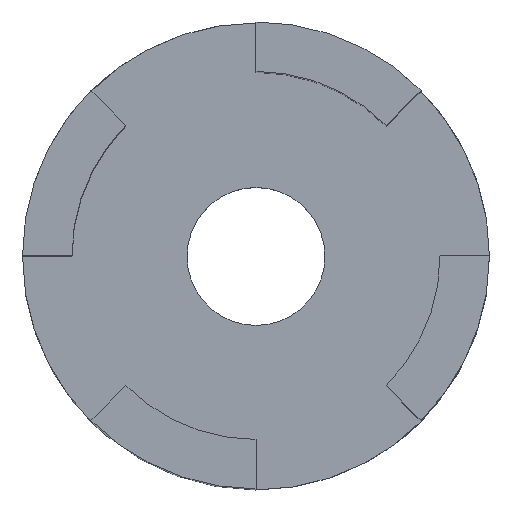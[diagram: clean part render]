
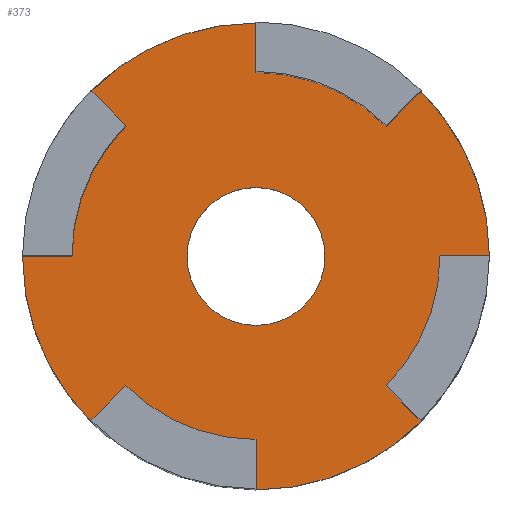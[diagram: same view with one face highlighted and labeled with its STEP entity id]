
A CAD part, top view. The second image highlights one B-rep face of the part: STEP entity #373.
In plain terms, the highlighted planar face has unit normal (0, 0, 1).
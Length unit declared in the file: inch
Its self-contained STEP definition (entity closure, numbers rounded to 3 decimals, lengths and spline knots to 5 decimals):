
#15=FACE_BOUND('',#65,.T.);
#26=PLANE('',#424);
#44=FACE_OUTER_BOUND('',#64,.T.);
#64=EDGE_LOOP('',(#300,#301,#302,#303,#304,#305,#306,#307,#308,#309,#310,
#311,#312,#313,#314,#315));
#65=EDGE_LOOP('',(#316));
#74=LINE('',#563,#108);
#79=LINE('',#577,#113);
#82=LINE('',#586,#116);
#87=LINE('',#600,#121);
#90=LINE('',#609,#124);
#95=LINE('',#623,#129);
#98=LINE('',#633,#132);
#99=LINE('',#637,#133);
#108=VECTOR('',#450,0.3937);
#113=VECTOR('',#463,0.3937);
#116=VECTOR('',#472,0.3937);
#121=VECTOR('',#485,0.3937);
#124=VECTOR('',#494,0.3937);
#129=VECTOR('',#507,0.3937);
#132=VECTOR('',#518,0.3937);
#133=VECTOR('',#521,0.3937);
#142=CIRCLE('',#402,0.11821);
#143=CIRCLE('',#405,0.31535);
#146=CIRCLE('',#412,0.31535);
#149=CIRCLE('',#419,0.31535);
#152=CIRCLE('',#425,0.4);
#153=CIRCLE('',#426,0.31535);
#154=CIRCLE('',#427,0.4);
#155=CIRCLE('',#428,0.4);
#156=CIRCLE('',#429,0.4);
#161=VERTEX_POINT('',#557);
#162=VERTEX_POINT('',#561);
#163=VERTEX_POINT('',#562);
#166=VERTEX_POINT('',#570);
#168=VERTEX_POINT('',#576);
#170=VERTEX_POINT('',#584);
#171=VERTEX_POINT('',#585);
#174=VERTEX_POINT('',#593);
#176=VERTEX_POINT('',#599);
#178=VERTEX_POINT('',#607);
#179=VERTEX_POINT('',#608);
#182=VERTEX_POINT('',#616);
#184=VERTEX_POINT('',#622);
#186=VERTEX_POINT('',#630);
#187=VERTEX_POINT('',#632);
#188=VERTEX_POINT('',#634);
#189=VERTEX_POINT('',#636);
#197=EDGE_CURVE('',#161,#161,#142,.T.);
#198=EDGE_CURVE('',#162,#163,#74,.T.);
#202=EDGE_CURVE('',#163,#166,#143,.T.);
#205=EDGE_CURVE('',#166,#168,#79,.T.);
#209=EDGE_CURVE('',#170,#171,#82,.T.);
#213=EDGE_CURVE('',#171,#174,#146,.T.);
#216=EDGE_CURVE('',#174,#176,#87,.T.);
#220=EDGE_CURVE('',#178,#179,#90,.T.);
#224=EDGE_CURVE('',#179,#182,#149,.T.);
#227=EDGE_CURVE('',#182,#184,#95,.T.);
#231=EDGE_CURVE('',#168,#186,#152,.T.);
#232=EDGE_CURVE('',#186,#187,#98,.T.);
#233=EDGE_CURVE('',#187,#188,#153,.T.);
#234=EDGE_CURVE('',#188,#189,#99,.T.);
#235=EDGE_CURVE('',#189,#178,#154,.T.);
#236=EDGE_CURVE('',#184,#170,#155,.T.);
#237=EDGE_CURVE('',#176,#162,#156,.T.);
#300=ORIENTED_EDGE('',*,*,#198,.T.);
#301=ORIENTED_EDGE('',*,*,#202,.T.);
#302=ORIENTED_EDGE('',*,*,#205,.T.);
#303=ORIENTED_EDGE('',*,*,#231,.T.);
#304=ORIENTED_EDGE('',*,*,#232,.T.);
#305=ORIENTED_EDGE('',*,*,#233,.T.);
#306=ORIENTED_EDGE('',*,*,#234,.T.);
#307=ORIENTED_EDGE('',*,*,#235,.T.);
#308=ORIENTED_EDGE('',*,*,#220,.T.);
#309=ORIENTED_EDGE('',*,*,#224,.T.);
#310=ORIENTED_EDGE('',*,*,#227,.T.);
#311=ORIENTED_EDGE('',*,*,#236,.T.);
#312=ORIENTED_EDGE('',*,*,#209,.T.);
#313=ORIENTED_EDGE('',*,*,#213,.T.);
#314=ORIENTED_EDGE('',*,*,#216,.T.);
#315=ORIENTED_EDGE('',*,*,#237,.T.);
#316=ORIENTED_EDGE('',*,*,#197,.T.);
#373=ADVANCED_FACE('',(#44,#15),#26,.T.);
#402=AXIS2_PLACEMENT_3D('',#559,#446,#447);
#405=AXIS2_PLACEMENT_3D('',#571,#456,#457);
#412=AXIS2_PLACEMENT_3D('',#594,#478,#479);
#419=AXIS2_PLACEMENT_3D('',#617,#500,#501);
#424=AXIS2_PLACEMENT_3D('',#629,#514,#515);
#425=AXIS2_PLACEMENT_3D('',#631,#516,#517);
#426=AXIS2_PLACEMENT_3D('',#635,#519,#520);
#427=AXIS2_PLACEMENT_3D('',#638,#522,#523);
#428=AXIS2_PLACEMENT_3D('',#639,#524,#525);
#429=AXIS2_PLACEMENT_3D('',#640,#526,#527);
#446=DIRECTION('center_axis',(0.,0.,-1.));
#447=DIRECTION('ref_axis',(-1.,0.,0.));
#450=DIRECTION('',(0.707,0.707,0.));
#456=DIRECTION('center_axis',(0.,0.,1.));
#457=DIRECTION('ref_axis',(0.707,0.707,0.));
#463=DIRECTION('',(0.,-1.,0.));
#472=DIRECTION('',(0.707,-0.707,0.));
#478=DIRECTION('center_axis',(0.,0.,1.));
#479=DIRECTION('ref_axis',(0.707,-0.707,0.));
#485=DIRECTION('',(-1.,0.,0.));
#494=DIRECTION('',(-0.707,-0.707,0.));
#500=DIRECTION('center_axis',(0.,0.,1.));
#501=DIRECTION('ref_axis',(-0.707,-0.707,0.));
#507=DIRECTION('',(0.,1.,0.));
#514=DIRECTION('center_axis',(0.,0.,1.));
#515=DIRECTION('ref_axis',(1.,0.,0.));
#516=DIRECTION('center_axis',(0.,0.,1.));
#517=DIRECTION('ref_axis',(1.,0.,0.));
#518=DIRECTION('',(-0.707,0.707,0.));
#519=DIRECTION('center_axis',(0.,0.,1.));
#520=DIRECTION('ref_axis',(-0.707,0.707,0.));
#521=DIRECTION('',(1.,0.,0.));
#522=DIRECTION('center_axis',(0.,0.,1.));
#523=DIRECTION('ref_axis',(1.,0.,0.));
#524=DIRECTION('center_axis',(0.,0.,1.));
#525=DIRECTION('ref_axis',(1.,0.,0.));
#526=DIRECTION('center_axis',(0.,0.,1.));
#527=DIRECTION('ref_axis',(1.,0.,0.));
#557=CARTESIAN_POINT('',(0.11821,0.,0.1));
#559=CARTESIAN_POINT('Origin',(0.,0.,0.1));
#561=CARTESIAN_POINT('',(-0.28284,-0.28284,0.1));
#562=CARTESIAN_POINT('',(-0.22299,-0.22299,0.1));
#563=CARTESIAN_POINT('',(-0.11149,-0.11149,0.1));
#570=CARTESIAN_POINT('',(0.,-0.31535,0.1));
#571=CARTESIAN_POINT('Origin',(0.,0.,
0.1));
#576=CARTESIAN_POINT('',(0.,-0.4,0.1));
#577=CARTESIAN_POINT('',(0.,-0.2,0.1));
#584=CARTESIAN_POINT('',(-0.28284,0.28284,0.1));
#585=CARTESIAN_POINT('',(-0.22299,0.22299,0.1));
#586=CARTESIAN_POINT('',(-0.11149,0.11149,0.1));
#593=CARTESIAN_POINT('',(-0.31535,0.,0.1));
#594=CARTESIAN_POINT('Origin',(0.,0.,
0.1));
#599=CARTESIAN_POINT('',(-0.4,0.,0.1));
#600=CARTESIAN_POINT('',(-0.2,0.,0.1));
#607=CARTESIAN_POINT('',(0.28284,0.28284,0.1));
#608=CARTESIAN_POINT('',(0.22299,0.22299,0.1));
#609=CARTESIAN_POINT('',(0.11149,0.11149,0.1));
#616=CARTESIAN_POINT('',(0.,0.31535,0.1));
#617=CARTESIAN_POINT('Origin',(0.,0.,
0.1));
#622=CARTESIAN_POINT('',(0.,0.4,0.1));
#623=CARTESIAN_POINT('',(0.,0.2,0.1));
#629=CARTESIAN_POINT('Origin',(0.,0.,
0.1));
#630=CARTESIAN_POINT('',(0.28284,-0.28284,0.1));
#631=CARTESIAN_POINT('Origin',(0.,0.,0.1));
#632=CARTESIAN_POINT('',(0.22299,-0.22299,0.1));
#633=CARTESIAN_POINT('',(0.11149,-0.11149,0.1));
#634=CARTESIAN_POINT('',(0.31535,0.,0.1));
#635=CARTESIAN_POINT('Origin',(0.,0.,
0.1));
#636=CARTESIAN_POINT('',(0.4,0.,0.1));
#637=CARTESIAN_POINT('',(0.2,0.,0.1));
#638=CARTESIAN_POINT('Origin',(0.,0.,0.1));
#639=CARTESIAN_POINT('Origin',(0.,0.,0.1));
#640=CARTESIAN_POINT('Origin',(0.,0.,0.1));
